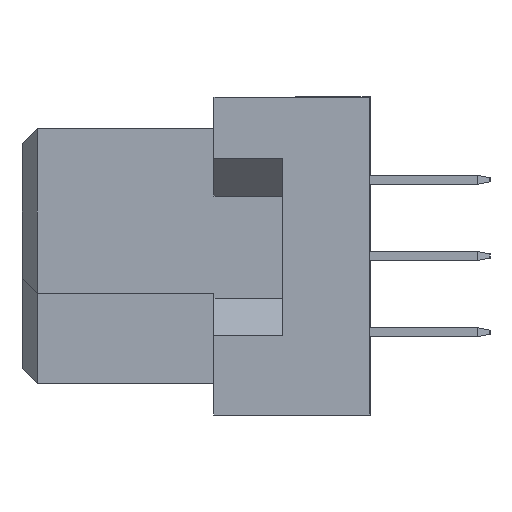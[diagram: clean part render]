
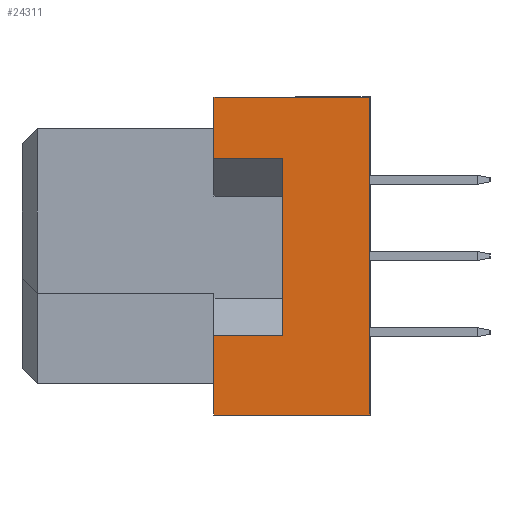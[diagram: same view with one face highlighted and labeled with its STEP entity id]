
A CAD part, left-side view. The second image highlights one B-rep face of the part: STEP entity #24311.
In plain terms, the highlighted planar face has unit normal (-1, 0, 0).
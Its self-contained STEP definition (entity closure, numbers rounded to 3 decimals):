
#967 = DIRECTION ( 'NONE',  ( 0., 0., 1. ) ) ;
#2516 = EDGE_CURVE ( 'NONE', #37028, #30869, #7898, .T. ) ;
#2540 = ORIENTED_EDGE ( 'NONE', *, *, #30992, .F. ) ;
#3791 = VERTEX_POINT ( 'NONE', #14322 ) ;
#4432 = CARTESIAN_POINT ( 'NONE',  ( -47.5, -6.4, -2.65 ) ) ;
#5795 = CARTESIAN_POINT ( 'NONE',  ( -47.5, -11.6, -5.3 ) ) ;
#7436 = DIRECTION ( 'NONE',  ( 0., 0., 1. ) ) ;
#7898 = LINE ( 'NONE', #29171, #28408 ) ;
#8515 = VERTEX_POINT ( 'NONE', #22157 ) ;
#8939 = CARTESIAN_POINT ( 'NONE',  ( -47.5, -8.7, -2.65 ) ) ;
#10417 = VERTEX_POINT ( 'NONE', #4432 ) ;
#10743 = LINE ( 'NONE', #20456, #24790 ) ;
#11042 = AXIS2_PLACEMENT_3D ( 'NONE', #23140, #26248, #7436 ) ;
#11065 = CARTESIAN_POINT ( 'NONE',  ( -47.5, -8.7, -2.65 ) ) ;
#11998 = LINE ( 'NONE', #5795, #16762 ) ;
#12045 = DIRECTION ( 'NONE',  ( 0., 0., 1. ) ) ;
#13014 = ORIENTED_EDGE ( 'NONE', *, *, #25265, .F. ) ;
#14322 = CARTESIAN_POINT ( 'NONE',  ( -47.5, -11.6, -5.3 ) ) ;
#14371 = DIRECTION ( 'NONE',  ( 0., 0., 1. ) ) ;
#15101 = DIRECTION ( 'NONE',  ( 0., 1., 0. ) ) ;
#16762 = VECTOR ( 'NONE', #15101, 1000. ) ;
#16906 = EDGE_LOOP ( 'NONE', ( #18183, #36399, #2540, #35366, #40299, #13014, #37474, #29250 ) ) ;
#17351 = PLANE ( 'NONE',  #11042 ) ;
#17382 = CARTESIAN_POINT ( 'NONE',  ( -47.5, -8.7, -2.65 ) ) ;
#18183 = ORIENTED_EDGE ( 'NONE', *, *, #20068, .T. ) ;
#19194 = VERTEX_POINT ( 'NONE', #36541 ) ;
#20068 = EDGE_CURVE ( 'NONE', #32188, #10417, #23442, .T. ) ;
#20456 = CARTESIAN_POINT ( 'NONE',  ( -47.5, -11.6, 5.3 ) ) ;
#20505 = DIRECTION ( 'NONE',  ( 0., 1., 0. ) ) ;
#20655 = VECTOR ( 'NONE', #967, 1000. ) ;
#21517 = DIRECTION ( 'NONE',  ( 0., 0., 1. ) ) ;
#21904 = LINE ( 'NONE', #34107, #30744 ) ;
#22157 = CARTESIAN_POINT ( 'NONE',  ( -47.5, -6.4, 5.3 ) ) ;
#22766 = EDGE_CURVE ( 'NONE', #19194, #10417, #21904, .T. ) ;
#23093 = EDGE_CURVE ( 'NONE', #27622, #8515, #10743, .T. ) ;
#23140 = CARTESIAN_POINT ( 'NONE',  ( -47.5, -11.6, 5.3 ) ) ;
#23362 = CARTESIAN_POINT ( 'NONE',  ( -47.5, -11.6, 5.3 ) ) ;
#23442 = LINE ( 'NONE', #11065, #36623 ) ;
#23656 = LINE ( 'NONE', #38935, #28200 ) ;
#24311 = ADVANCED_FACE ( 'NONE', ( #34713 ), #17351, .T. ) ;
#24790 = VECTOR ( 'NONE', #32625, 1000. ) ;
#25265 = EDGE_CURVE ( 'NONE', #30869, #8515, #23656, .T. ) ;
#25521 = CARTESIAN_POINT ( 'NONE',  ( -47.5, -8.7, 3.25 ) ) ;
#25965 = LINE ( 'NONE', #28857, #20655 ) ;
#26248 = DIRECTION ( 'NONE',  ( -1., 0., 0. ) ) ;
#26332 = DIRECTION ( 'NONE',  ( 0., 1., 0. ) ) ;
#26534 = VECTOR ( 'NONE', #12045, 1000. ) ;
#27622 = VERTEX_POINT ( 'NONE', #23362 ) ;
#28200 = VECTOR ( 'NONE', #14371, 1000. ) ;
#28408 = VECTOR ( 'NONE', #20505, 1000. ) ;
#28473 = EDGE_CURVE ( 'NONE', #32188, #37028, #35656, .T. ) ;
#28857 = CARTESIAN_POINT ( 'NONE',  ( -47.5, -11.6, 5.3 ) ) ;
#29171 = CARTESIAN_POINT ( 'NONE',  ( -47.5, -8.7, 3.25 ) ) ;
#29250 = ORIENTED_EDGE ( 'NONE', *, *, #28473, .F. ) ;
#29688 = EDGE_CURVE ( 'NONE', #3791, #27622, #25965, .T. ) ;
#29963 = CARTESIAN_POINT ( 'NONE',  ( -47.5, -6.4, 3.25 ) ) ;
#30744 = VECTOR ( 'NONE', #21517, 1000. ) ;
#30869 = VERTEX_POINT ( 'NONE', #29963 ) ;
#30992 = EDGE_CURVE ( 'NONE', #3791, #19194, #11998, .T. ) ;
#32188 = VERTEX_POINT ( 'NONE', #17382 ) ;
#32625 = DIRECTION ( 'NONE',  ( 0., 1., 0. ) ) ;
#34107 = CARTESIAN_POINT ( 'NONE',  ( -47.5, -6.4, -5.3 ) ) ;
#34713 = FACE_OUTER_BOUND ( 'NONE', #16906, .T. ) ;
#35366 = ORIENTED_EDGE ( 'NONE', *, *, #29688, .T. ) ;
#35656 = LINE ( 'NONE', #8939, #26534 ) ;
#36399 = ORIENTED_EDGE ( 'NONE', *, *, #22766, .F. ) ;
#36541 = CARTESIAN_POINT ( 'NONE',  ( -47.5, -6.4, -5.3 ) ) ;
#36623 = VECTOR ( 'NONE', #26332, 1000. ) ;
#37028 = VERTEX_POINT ( 'NONE', #25521 ) ;
#37474 = ORIENTED_EDGE ( 'NONE', *, *, #2516, .F. ) ;
#38935 = CARTESIAN_POINT ( 'NONE',  ( -47.5, -6.4, -5.3 ) ) ;
#40299 = ORIENTED_EDGE ( 'NONE', *, *, #23093, .T. ) ;
